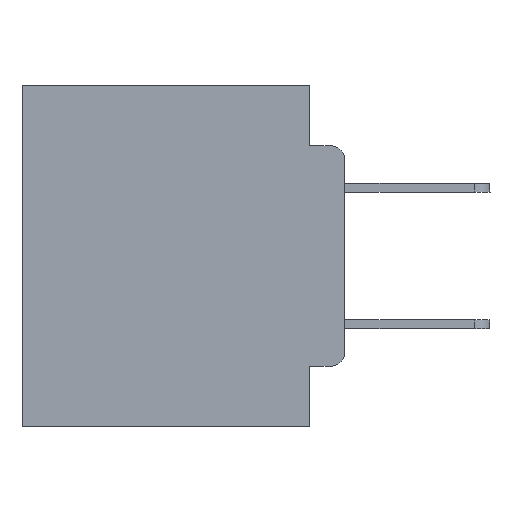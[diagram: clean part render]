
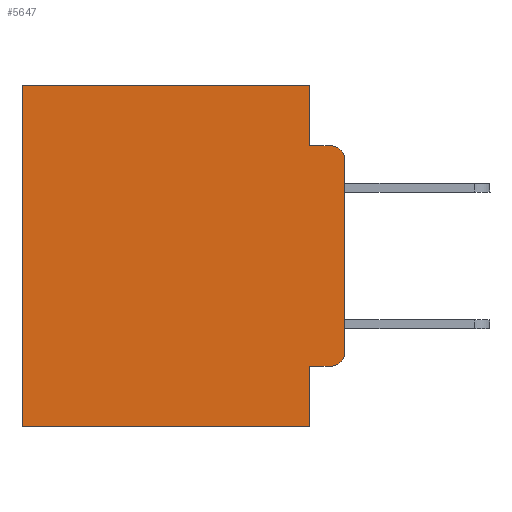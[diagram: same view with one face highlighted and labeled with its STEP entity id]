
A CAD part, left-side view. The second image highlights one B-rep face of the part: STEP entity #5647.
In plain terms, the highlighted planar face has unit normal (-1, 0, 0).
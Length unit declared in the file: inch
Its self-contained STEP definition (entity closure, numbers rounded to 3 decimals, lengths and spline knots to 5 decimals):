
#681 = CARTESIAN_POINT ( 'NONE',  ( 0.298, 0.02, -0.1085 ) ) ;
#777 = CARTESIAN_POINT ( 'NONE',  ( 0.298, 0.051, -0.5 ) ) ;
#949 = CARTESIAN_POINT ( 'NONE',  ( 0.298, 0.051, -0.4115 ) ) ;
#1620 = DIRECTION ( 'NONE',  ( 0., 0., -1. ) ) ;
#2774 = DIRECTION ( 'NONE',  ( 0., 0., -1. ) ) ;
#3255 = ORIENTED_EDGE ( 'NONE', *, *, #13269, .F. ) ;
#4553 = EDGE_CURVE ( 'NONE', #8115, #10714, #6472, .T. ) ;
#5289 = CARTESIAN_POINT ( 'NONE',  ( 0.298, 0., -0.1085 ) ) ;
#5457 = CARTESIAN_POINT ( 'NONE',  ( 0.298, 0., 0. ) ) ;
#5647 = ADVANCED_FACE ( 'NONE', ( #7694 ), #19031, .F. ) ;
#5700 = CARTESIAN_POINT ( 'NONE',  ( 0.298, 0.473, 0. ) ) ;
#6377 = VECTOR ( 'NONE', #6490, 39.37008 ) ;
#6444 = LINE ( 'NONE', #23263, #7800 ) ;
#6472 = LINE ( 'NONE', #17956, #12291 ) ;
#6490 = DIRECTION ( 'NONE',  ( 0., 0., -1. ) ) ;
#6491 = ORIENTED_EDGE ( 'NONE', *, *, #6546, .T. ) ;
#6496 = EDGE_CURVE ( 'NONE', #24671, #24473, #6444, .T. ) ;
#6512 = VERTEX_POINT ( 'NONE', #777 ) ;
#6546 = EDGE_CURVE ( 'NONE', #25746, #26209, #25447, .T. ) ;
#6627 = AXIS2_PLACEMENT_3D ( 'NONE', #5457, #9642, #23776 ) ;
#6636 = CARTESIAN_POINT ( 'NONE',  ( 0.298, 0., -0.5 ) ) ;
#6941 = DIRECTION ( 'NONE',  ( 0., 1., 0. ) ) ;
#7054 = LINE ( 'NONE', #24531, #6377 ) ;
#7563 = ORIENTED_EDGE ( 'NONE', *, *, #22193, .F. ) ;
#7595 = VECTOR ( 'NONE', #14648, 39.37008 ) ;
#7694 = FACE_OUTER_BOUND ( 'NONE', #28581, .T. ) ;
#7703 = CARTESIAN_POINT ( 'NONE',  ( 0.298, 0., 0. ) ) ;
#7748 = VECTOR ( 'NONE', #8997, 39.37008 ) ;
#7800 = VECTOR ( 'NONE', #25500, 39.37008 ) ;
#8115 = VERTEX_POINT ( 'NONE', #5700 ) ;
#8153 = VECTOR ( 'NONE', #1620, 39.37008 ) ;
#8161 = CARTESIAN_POINT ( 'NONE',  ( 0.298, 0.051, 0. ) ) ;
#8997 = DIRECTION ( 'NONE',  ( 0., -1., 0. ) ) ;
#9413 = EDGE_CURVE ( 'NONE', #6512, #10714, #18270, .T. ) ;
#9642 = DIRECTION ( 'NONE',  ( 1., 0., 0. ) ) ;
#10306 = CARTESIAN_POINT ( 'NONE',  ( 0.298, 0.02, -0.4115 ) ) ;
#10351 = VERTEX_POINT ( 'NONE', #16059 ) ;
#10714 = VERTEX_POINT ( 'NONE', #23156 ) ;
#11930 = AXIS2_PLACEMENT_3D ( 'NONE', #681, #23158, #2774 ) ;
#12103 = EDGE_CURVE ( 'NONE', #15247, #28730, #14788, .T. ) ;
#12291 = VECTOR ( 'NONE', #28948, 39.37008 ) ;
#12406 = ORIENTED_EDGE ( 'NONE', *, *, #20953, .F. ) ;
#13269 = EDGE_CURVE ( 'NONE', #25746, #6512, #22304, .T. ) ;
#13387 = CARTESIAN_POINT ( 'NONE',  ( 0.298, 0.051, 0. ) ) ;
#13906 = LINE ( 'NONE', #29216, #7748 ) ;
#14648 = DIRECTION ( 'NONE',  ( 0., -1., 0. ) ) ;
#14788 = CIRCLE ( 'NONE', #11930, 0.02 ) ;
#14793 = ORIENTED_EDGE ( 'NONE', *, *, #9413, .F. ) ;
#15247 = VERTEX_POINT ( 'NONE', #5289 ) ;
#15601 = DIRECTION ( 'NONE',  ( 0., 0., -1. ) ) ;
#16059 = CARTESIAN_POINT ( 'NONE',  ( 0.298, 0., -0.3915 ) ) ;
#16641 = DIRECTION ( 'NONE',  ( 0., 1., 0. ) ) ;
#17333 = CARTESIAN_POINT ( 'NONE',  ( 0.298, 0.051, -0.4115 ) ) ;
#17538 = ORIENTED_EDGE ( 'NONE', *, *, #18769, .T. ) ;
#17956 = CARTESIAN_POINT ( 'NONE',  ( 0.298, 0.473, 0. ) ) ;
#18059 = VECTOR ( 'NONE', #6941, 39.37008 ) ;
#18270 = LINE ( 'NONE', #6636, #18059 ) ;
#18451 = VECTOR ( 'NONE', #16641, 39.37008 ) ;
#18769 = EDGE_CURVE ( 'NONE', #26209, #10351, #20221, .T. ) ;
#19031 = PLANE ( 'NONE',  #6627 ) ;
#20221 = CIRCLE ( 'NONE', #24981, 0.02 ) ;
#20224 = EDGE_CURVE ( 'NONE', #24671, #8115, #28385, .T. ) ;
#20678 = CARTESIAN_POINT ( 'NONE',  ( 0.298, 0.051, -0.0885 ) ) ;
#20953 = EDGE_CURVE ( 'NONE', #24473, #28730, #13906, .T. ) ;
#21179 = ORIENTED_EDGE ( 'NONE', *, *, #6496, .F. ) ;
#22193 = EDGE_CURVE ( 'NONE', #15247, #10351, #7054, .T. ) ;
#22205 = ORIENTED_EDGE ( 'NONE', *, *, #12103, .T. ) ;
#22304 = LINE ( 'NONE', #13387, #8153 ) ;
#22996 = CARTESIAN_POINT ( 'NONE',  ( 0.298, 0.02, -0.0885 ) ) ;
#23156 = CARTESIAN_POINT ( 'NONE',  ( 0.298, 0.473, -0.5 ) ) ;
#23158 = DIRECTION ( 'NONE',  ( -1., 0., 0. ) ) ;
#23263 = CARTESIAN_POINT ( 'NONE',  ( 0.298, 0.051, 0. ) ) ;
#23776 = DIRECTION ( 'NONE',  ( 0., 0., -1. ) ) ;
#24473 = VERTEX_POINT ( 'NONE', #20678 ) ;
#24531 = CARTESIAN_POINT ( 'NONE',  ( 0.298, 0., 0. ) ) ;
#24671 = VERTEX_POINT ( 'NONE', #8161 ) ;
#24981 = AXIS2_PLACEMENT_3D ( 'NONE', #28698, #29129, #15601 ) ;
#25447 = LINE ( 'NONE', #949, #7595 ) ;
#25500 = DIRECTION ( 'NONE',  ( 0., 0., -1. ) ) ;
#25746 = VERTEX_POINT ( 'NONE', #17333 ) ;
#26209 = VERTEX_POINT ( 'NONE', #10306 ) ;
#27385 = ORIENTED_EDGE ( 'NONE', *, *, #4553, .T. ) ;
#28385 = LINE ( 'NONE', #7703, #18451 ) ;
#28581 = EDGE_LOOP ( 'NONE', ( #7563, #22205, #12406, #21179, #28594, #27385, #14793, #3255, #6491, #17538 ) ) ;
#28594 = ORIENTED_EDGE ( 'NONE', *, *, #20224, .T. ) ;
#28698 = CARTESIAN_POINT ( 'NONE',  ( 0.298, 0.02, -0.3915 ) ) ;
#28730 = VERTEX_POINT ( 'NONE', #22996 ) ;
#28948 = DIRECTION ( 'NONE',  ( 0., 0., -1. ) ) ;
#29129 = DIRECTION ( 'NONE',  ( -1., 0., 0. ) ) ;
#29216 = CARTESIAN_POINT ( 'NONE',  ( 0.298, 0.051, -0.0885 ) ) ;
